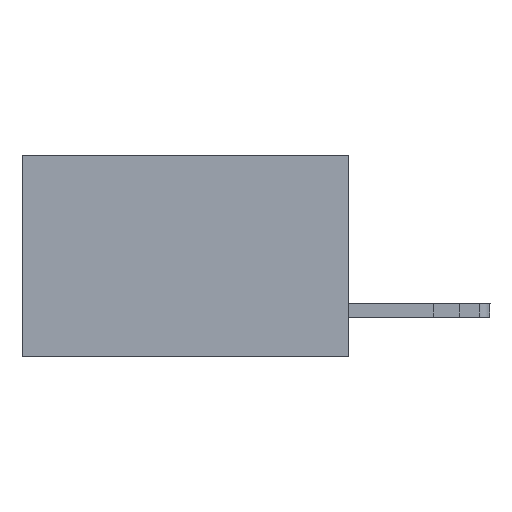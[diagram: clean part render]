
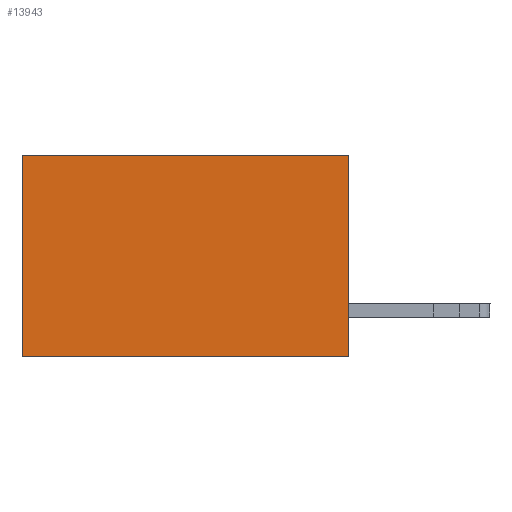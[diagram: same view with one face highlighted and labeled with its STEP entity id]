
A CAD part, left-side view. The second image highlights one B-rep face of the part: STEP entity #13943.
In plain terms, the highlighted planar face has unit normal (-1, 0, 0).
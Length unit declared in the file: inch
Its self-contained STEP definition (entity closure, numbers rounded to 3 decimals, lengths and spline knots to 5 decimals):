
#146 = ORIENTED_EDGE ( 'NONE', *, *, #9382, .T. ) ;
#321 = VERTEX_POINT ( 'NONE', #9292 ) ;
#405 = LINE ( 'NONE', #9905, #14809 ) ;
#475 = LINE ( 'NONE', #8031, #9668 ) ;
#698 = DIRECTION ( 'NONE',  ( 0., 1., 0. ) ) ;
#784 = ORIENTED_EDGE ( 'NONE', *, *, #14827, .F. ) ;
#968 = VECTOR ( 'NONE', #698, 39.37008 ) ;
#1367 = DIRECTION ( 'NONE',  ( 0., 0., -1. ) ) ;
#1809 = CARTESIAN_POINT ( 'NONE',  ( 0.298, 0., -0.37 ) ) ;
#2391 = CARTESIAN_POINT ( 'NONE',  ( 0.298, 0.6, -0.37 ) ) ;
#2439 = CARTESIAN_POINT ( 'NONE',  ( 0.298, 0., -0.37 ) ) ;
#3020 = ORIENTED_EDGE ( 'NONE', *, *, #8893, .F. ) ;
#4466 = LINE ( 'NONE', #7152, #6831 ) ;
#6532 = DIRECTION ( 'NONE',  ( 0., 1., 0. ) ) ;
#6831 = VECTOR ( 'NONE', #1367, 39.37008 ) ;
#7118 = LINE ( 'NONE', #1809, #968 ) ;
#7152 = CARTESIAN_POINT ( 'NONE',  ( 0.298, 0.6, 0. ) ) ;
#7914 = FACE_OUTER_BOUND ( 'NONE', #11106, .T. ) ;
#8031 = CARTESIAN_POINT ( 'NONE',  ( 0.298, 0., 0. ) ) ;
#8144 = VERTEX_POINT ( 'NONE', #9363 ) ;
#8893 = EDGE_CURVE ( 'NONE', #11870, #12603, #7118, .T. ) ;
#9292 = CARTESIAN_POINT ( 'NONE',  ( 0.298, 0.6, 0. ) ) ;
#9363 = CARTESIAN_POINT ( 'NONE',  ( 0.298, 0., 0. ) ) ;
#9382 = EDGE_CURVE ( 'NONE', #8144, #321, #405, .T. ) ;
#9668 = VECTOR ( 'NONE', #11331, 39.37008 ) ;
#9905 = CARTESIAN_POINT ( 'NONE',  ( 0.298, 0., 0. ) ) ;
#10247 = DIRECTION ( 'NONE',  ( 1., 0., 0. ) ) ;
#11106 = EDGE_LOOP ( 'NONE', ( #13730, #3020, #784, #146 ) ) ;
#11331 = DIRECTION ( 'NONE',  ( 0., 0., -1. ) ) ;
#11347 = DIRECTION ( 'NONE',  ( 0., 0., -1. ) ) ;
#11870 = VERTEX_POINT ( 'NONE', #2439 ) ;
#12511 = PLANE ( 'NONE',  #14401 ) ;
#12603 = VERTEX_POINT ( 'NONE', #2391 ) ;
#12623 = CARTESIAN_POINT ( 'NONE',  ( 0.298, 0., 0. ) ) ;
#13577 = EDGE_CURVE ( 'NONE', #321, #12603, #4466, .T. ) ;
#13730 = ORIENTED_EDGE ( 'NONE', *, *, #13577, .T. ) ;
#13943 = ADVANCED_FACE ( 'NONE', ( #7914 ), #12511, .F. ) ;
#14401 = AXIS2_PLACEMENT_3D ( 'NONE', #12623, #10247, #11347 ) ;
#14809 = VECTOR ( 'NONE', #6532, 39.37008 ) ;
#14827 = EDGE_CURVE ( 'NONE', #8144, #11870, #475, .T. ) ;
